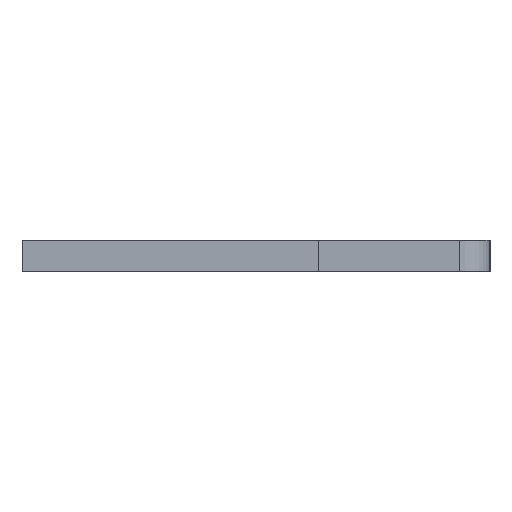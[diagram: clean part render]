
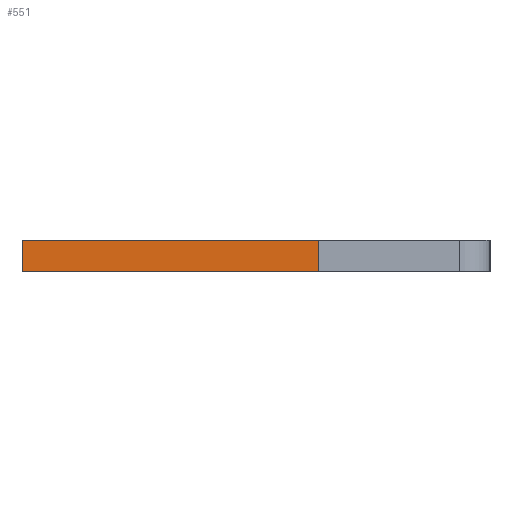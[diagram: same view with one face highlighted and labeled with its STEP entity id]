
A CAD part, left-side view. The second image highlights one B-rep face of the part: STEP entity #551.
In plain terms, the highlighted face is planar.
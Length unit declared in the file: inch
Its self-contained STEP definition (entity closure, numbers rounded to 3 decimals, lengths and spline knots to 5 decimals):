
#27 = VERTEX_POINT ( 'NONE', #1102 ) ;
#53 = CARTESIAN_POINT ( 'NONE',  ( -0.01, 0.15, -0.04 ) ) ;
#63 = EDGE_CURVE ( 'NONE', #403, #448, #865, .T. ) ;
#77 = FACE_OUTER_BOUND ( 'NONE', #916, .T. ) ;
#108 = CARTESIAN_POINT ( 'NONE',  ( 0.01, 0.15, -0.04 ) ) ;
#158 = DIRECTION ( 'NONE',  ( 1., 0., 0. ) ) ;
#164 = CARTESIAN_POINT ( 'NONE',  ( 0.01, 0.15, -0.04 ) ) ;
#200 = LINE ( 'NONE', #789, #1207 ) ;
#275 = VECTOR ( 'NONE', #605, 39.37008 ) ;
#276 = LINE ( 'NONE', #164, #804 ) ;
#301 = VERTEX_POINT ( 'NONE', #1032 ) ;
#308 = VECTOR ( 'NONE', #559, 39.37008 ) ;
#351 = CARTESIAN_POINT ( 'NONE',  ( 0.01, -0.04, -0.04 ) ) ;
#403 = VERTEX_POINT ( 'NONE', #533 ) ;
#447 = AXIS2_PLACEMENT_3D ( 'NONE', #743, #761, #158 ) ;
#448 = VERTEX_POINT ( 'NONE', #53 ) ;
#533 = CARTESIAN_POINT ( 'NONE',  ( 0.01, 0.15, -0.04 ) ) ;
#551 = ADVANCED_FACE ( 'NONE', ( #77 ), #653, .F. ) ;
#555 = EDGE_CURVE ( 'NONE', #27, #301, #663, .T. ) ;
#559 = DIRECTION ( 'NONE',  ( -1., 0., 0. ) ) ;
#591 = EDGE_CURVE ( 'NONE', #27, #403, #276, .T. ) ;
#605 = DIRECTION ( 'NONE',  ( -1., 0., 0. ) ) ;
#653 = PLANE ( 'NONE',  #447 ) ;
#663 = LINE ( 'NONE', #351, #308 ) ;
#690 = DIRECTION ( 'NONE',  ( 0., 1., 0. ) ) ;
#743 = CARTESIAN_POINT ( 'NONE',  ( 0.01, 0.15, -0.04 ) ) ;
#761 = DIRECTION ( 'NONE',  ( 0., 0., 1. ) ) ;
#789 = CARTESIAN_POINT ( 'NONE',  ( -0.01, 0.15, -0.04 ) ) ;
#804 = VECTOR ( 'NONE', #855, 39.37008 ) ;
#855 = DIRECTION ( 'NONE',  ( 0., 1., 0. ) ) ;
#865 = LINE ( 'NONE', #108, #275 ) ;
#916 = EDGE_LOOP ( 'NONE', ( #922, #946, #1103, #1076 ) ) ;
#922 = ORIENTED_EDGE ( 'NONE', *, *, #1084, .T. ) ;
#946 = ORIENTED_EDGE ( 'NONE', *, *, #63, .F. ) ;
#1032 = CARTESIAN_POINT ( 'NONE',  ( -0.01, -0.04, -0.04 ) ) ;
#1076 = ORIENTED_EDGE ( 'NONE', *, *, #555, .T. ) ;
#1084 = EDGE_CURVE ( 'NONE', #301, #448, #200, .T. ) ;
#1102 = CARTESIAN_POINT ( 'NONE',  ( 0.01, -0.04, -0.04 ) ) ;
#1103 = ORIENTED_EDGE ( 'NONE', *, *, #591, .F. ) ;
#1207 = VECTOR ( 'NONE', #690, 39.37008 ) ;
